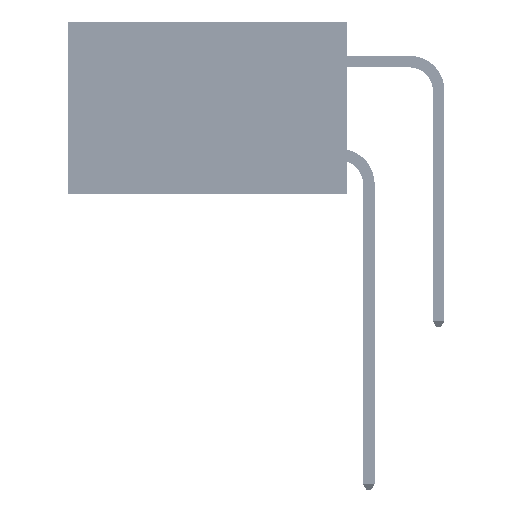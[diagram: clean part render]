
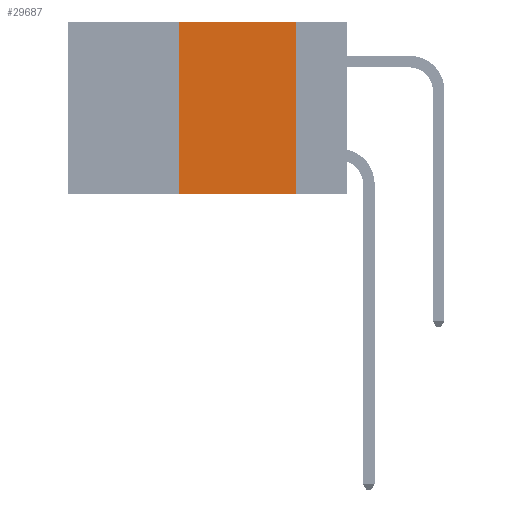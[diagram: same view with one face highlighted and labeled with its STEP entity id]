
A CAD part, left-side view. The second image highlights one B-rep face of the part: STEP entity #29687.
In plain terms, the highlighted planar face has unit normal (-1, 0, 0).
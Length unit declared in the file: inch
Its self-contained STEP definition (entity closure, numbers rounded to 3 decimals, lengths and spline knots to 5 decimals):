
#120 = EDGE_CURVE ( 'NONE', #1458, #2927, #22973, .T. ) ;
#285 = CARTESIAN_POINT ( 'NONE',  ( 0., 0.36, -0.37 ) ) ;
#999 = LINE ( 'NONE', #4468, #27243 ) ;
#1458 = VERTEX_POINT ( 'NONE', #285 ) ;
#2346 = CARTESIAN_POINT ( 'NONE',  ( 0., 0.6, 0. ) ) ;
#2489 = DIRECTION ( 'NONE',  ( 0., -1., 0. ) ) ;
#2821 = FACE_OUTER_BOUND ( 'NONE', #35406, .T. ) ;
#2927 = VERTEX_POINT ( 'NONE', #33727 ) ;
#3357 = CARTESIAN_POINT ( 'NONE',  ( 0., 0.36, 0. ) ) ;
#3925 = CARTESIAN_POINT ( 'NONE',  ( 0., 0.6, -0.37 ) ) ;
#4300 = VECTOR ( 'NONE', #18946, 39.37008 ) ;
#4399 = ORIENTED_EDGE ( 'NONE', *, *, #27960, .F. ) ;
#4468 = CARTESIAN_POINT ( 'NONE',  ( 0., 0.11, 0. ) ) ;
#6539 = DIRECTION ( 'NONE',  ( 1., 0., 0. ) ) ;
#7582 = VECTOR ( 'NONE', #2489, 39.37008 ) ;
#13635 = EDGE_CURVE ( 'NONE', #29813, #31626, #43072, .T. ) ;
#13718 = DIRECTION ( 'NONE',  ( 0., 0., -1. ) ) ;
#18946 = DIRECTION ( 'NONE',  ( 0., 0., 1. ) ) ;
#19080 = CARTESIAN_POINT ( 'NONE',  ( 0., 0.11, 0. ) ) ;
#19559 = DIRECTION ( 'NONE',  ( 0., 0., -1. ) ) ;
#20968 = VECTOR ( 'NONE', #42269, 39.37008 ) ;
#22973 = LINE ( 'NONE', #3925, #20968 ) ;
#24817 = AXIS2_PLACEMENT_3D ( 'NONE', #2346, #6539, #13718 ) ;
#27243 = VECTOR ( 'NONE', #19559, 39.37008 ) ;
#27960 = EDGE_CURVE ( 'NONE', #1458, #29813, #37242, .T. ) ;
#29687 = ADVANCED_FACE ( 'NONE', ( #2821 ), #48081, .F. ) ;
#29813 = VERTEX_POINT ( 'NONE', #45361 ) ;
#30365 = EDGE_CURVE ( 'NONE', #31626, #2927, #999, .T. ) ;
#31626 = VERTEX_POINT ( 'NONE', #19080 ) ;
#33727 = CARTESIAN_POINT ( 'NONE',  ( 0., 0.11, -0.37 ) ) ;
#35386 = ORIENTED_EDGE ( 'NONE', *, *, #120, .T. ) ;
#35406 = EDGE_LOOP ( 'NONE', ( #40639, #40953, #4399, #35386 ) ) ;
#37242 = LINE ( 'NONE', #3357, #4300 ) ;
#40639 = ORIENTED_EDGE ( 'NONE', *, *, #30365, .F. ) ;
#40953 = ORIENTED_EDGE ( 'NONE', *, *, #13635, .F. ) ;
#42269 = DIRECTION ( 'NONE',  ( 0., -1., 0. ) ) ;
#43072 = LINE ( 'NONE', #43565, #7582 ) ;
#43565 = CARTESIAN_POINT ( 'NONE',  ( 0., 0.6, 0. ) ) ;
#45361 = CARTESIAN_POINT ( 'NONE',  ( 0., 0.36, 0. ) ) ;
#48081 = PLANE ( 'NONE',  #24817 ) ;
